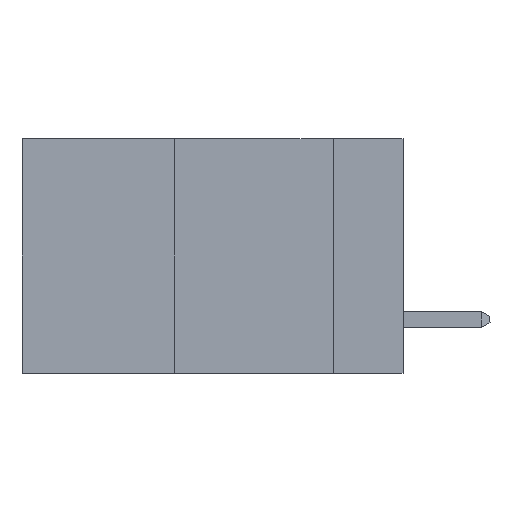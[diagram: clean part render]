
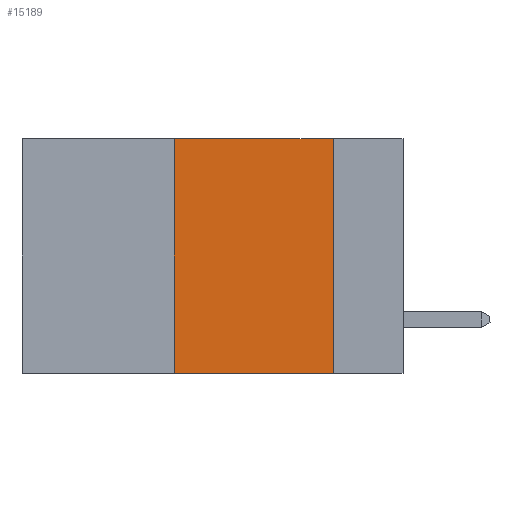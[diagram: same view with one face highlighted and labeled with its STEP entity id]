
A CAD part, left-side view. The second image highlights one B-rep face of the part: STEP entity #15189.
In plain terms, the highlighted planar face has unit normal (-1, 0, 0).
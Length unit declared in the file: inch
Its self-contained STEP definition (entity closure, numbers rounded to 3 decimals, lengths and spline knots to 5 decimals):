
#419 = CARTESIAN_POINT ( 'NONE',  ( 0., 0.6, 0. ) ) ;
#682 = VERTEX_POINT ( 'NONE', #12096 ) ;
#905 = CARTESIAN_POINT ( 'NONE',  ( 0., 0.11, 0. ) ) ;
#1380 = ORIENTED_EDGE ( 'NONE', *, *, #16810, .F. ) ;
#2763 = LINE ( 'NONE', #15483, #10635 ) ;
#3000 = LINE ( 'NONE', #419, #17427 ) ;
#3484 = VERTEX_POINT ( 'NONE', #6518 ) ;
#3654 = VERTEX_POINT ( 'NONE', #16953 ) ;
#3944 = EDGE_LOOP ( 'NONE', ( #4483, #16412, #1380, #13596 ) ) ;
#4213 = DIRECTION ( 'NONE',  ( 0., 0., -1. ) ) ;
#4483 = ORIENTED_EDGE ( 'NONE', *, *, #10828, .F. ) ;
#5428 = DIRECTION ( 'NONE',  ( 0., -1., 0. ) ) ;
#6518 = CARTESIAN_POINT ( 'NONE',  ( 0., 0.36, 0. ) ) ;
#8356 = CARTESIAN_POINT ( 'NONE',  ( 0., 0.36, 0. ) ) ;
#8666 = PLANE ( 'NONE',  #15594 ) ;
#8885 = VECTOR ( 'NONE', #10563, 39.37008 ) ;
#10563 = DIRECTION ( 'NONE',  ( 0., 0., -1. ) ) ;
#10635 = VECTOR ( 'NONE', #5428, 39.37008 ) ;
#10828 = EDGE_CURVE ( 'NONE', #17802, #682, #12727, .T. ) ;
#12096 = CARTESIAN_POINT ( 'NONE',  ( 0., 0.11, -0.37 ) ) ;
#12718 = DIRECTION ( 'NONE',  ( 0., 0., 1. ) ) ;
#12727 = LINE ( 'NONE', #16174, #8885 ) ;
#12955 = CARTESIAN_POINT ( 'NONE',  ( 0., 0.6, 0. ) ) ;
#13013 = DIRECTION ( 'NONE',  ( 1., 0., 0. ) ) ;
#13596 = ORIENTED_EDGE ( 'NONE', *, *, #16233, .T. ) ;
#14972 = DIRECTION ( 'NONE',  ( 0., -1., 0. ) ) ;
#15189 = ADVANCED_FACE ( 'NONE', ( #17468 ), #8666, .F. ) ;
#15265 = LINE ( 'NONE', #8356, #18470 ) ;
#15483 = CARTESIAN_POINT ( 'NONE',  ( 0., 0.6, -0.37 ) ) ;
#15594 = AXIS2_PLACEMENT_3D ( 'NONE', #12955, #13013, #4213 ) ;
#16174 = CARTESIAN_POINT ( 'NONE',  ( 0., 0.11, 0. ) ) ;
#16233 = EDGE_CURVE ( 'NONE', #3654, #682, #2763, .T. ) ;
#16412 = ORIENTED_EDGE ( 'NONE', *, *, #18650, .F. ) ;
#16810 = EDGE_CURVE ( 'NONE', #3654, #3484, #15265, .T. ) ;
#16953 = CARTESIAN_POINT ( 'NONE',  ( 0., 0.36, -0.37 ) ) ;
#17427 = VECTOR ( 'NONE', #14972, 39.37008 ) ;
#17468 = FACE_OUTER_BOUND ( 'NONE', #3944, .T. ) ;
#17802 = VERTEX_POINT ( 'NONE', #905 ) ;
#18470 = VECTOR ( 'NONE', #12718, 39.37008 ) ;
#18650 = EDGE_CURVE ( 'NONE', #3484, #17802, #3000, .T. ) ;
